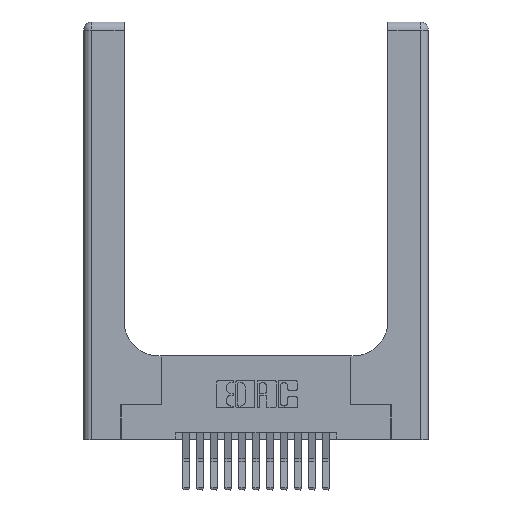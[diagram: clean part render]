
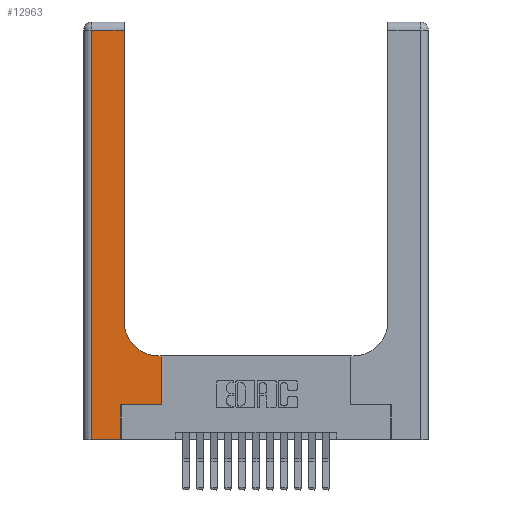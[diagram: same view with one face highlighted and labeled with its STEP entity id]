
A CAD part, top view. The second image highlights one B-rep face of the part: STEP entity #12963.
In plain terms, the highlighted planar face has unit normal (0, 0, 1).
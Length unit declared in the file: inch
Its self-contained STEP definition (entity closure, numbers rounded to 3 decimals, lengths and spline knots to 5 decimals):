
#119 = ORIENTED_EDGE ( 'NONE', *, *, #17524, .T. ) ;
#681 = ORIENTED_EDGE ( 'NONE', *, *, #6312, .T. ) ;
#894 = CARTESIAN_POINT ( 'NONE',  ( 0.5585, 0.6, 0.37 ) ) ;
#912 = LINE ( 'NONE', #16694, #14857 ) ;
#940 = EDGE_CURVE ( 'NONE', #12710, #9015, #12921, .T. ) ;
#1045 = AXIS2_PLACEMENT_3D ( 'NONE', #9175, #6428, #3822 ) ;
#1294 = EDGE_CURVE ( 'NONE', #9015, #9551, #13995, .T. ) ;
#1590 = CARTESIAN_POINT ( 'NONE',  ( 0.5415, 0.85, 0.37 ) ) ;
#1810 = LINE ( 'NONE', #12224, #9227 ) ;
#2588 = CARTESIAN_POINT ( 'NONE',  ( 0.5585, 0.25, 0.37 ) ) ;
#2897 = CARTESIAN_POINT ( 'NONE',  ( 0.2915, 2.94, 0.37 ) ) ;
#3028 = VECTOR ( 'NONE', #9323, 39.37008 ) ;
#3314 = CIRCLE ( 'NONE', #15575, 0.25 ) ;
#3367 = CARTESIAN_POINT ( 'NONE',  ( 0.5585, 0.25, 0.37 ) ) ;
#3822 = DIRECTION ( 'NONE',  ( -1., 0., 0. ) ) ;
#4126 = ORIENTED_EDGE ( 'NONE', *, *, #7134, .T. ) ;
#4908 = DIRECTION ( 'NONE',  ( 0., 1., 0. ) ) ;
#5151 = ORIENTED_EDGE ( 'NONE', *, *, #17037, .T. ) ;
#5170 = ORIENTED_EDGE ( 'NONE', *, *, #13499, .T. ) ;
#5340 = LINE ( 'NONE', #11966, #11842 ) ;
#5417 = DIRECTION ( 'NONE',  ( -1., 0., 0. ) ) ;
#5501 = ORIENTED_EDGE ( 'NONE', *, *, #17718, .T. ) ;
#5720 = ORIENTED_EDGE ( 'NONE', *, *, #14791, .T. ) ;
#6036 = CARTESIAN_POINT ( 'NONE',  ( 0.06, 2.94, 0.37 ) ) ;
#6074 = DIRECTION ( 'NONE',  ( 1., 0., 0. ) ) ;
#6312 = EDGE_CURVE ( 'NONE', #15978, #18007, #1810, .T. ) ;
#6428 = DIRECTION ( 'NONE',  ( 0., 0., -1. ) ) ;
#6876 = VECTOR ( 'NONE', #13115, 39.37008 ) ;
#7134 = EDGE_CURVE ( 'NONE', #9644, #15978, #3314, .T. ) ;
#7175 = DIRECTION ( 'NONE',  ( 1., 0., 0. ) ) ;
#7241 = CARTESIAN_POINT ( 'NONE',  ( 0.269, 0., 0.37 ) ) ;
#7255 = ORIENTED_EDGE ( 'NONE', *, *, #1294, .T. ) ;
#7330 = VERTEX_POINT ( 'NONE', #7241 ) ;
#8597 = VECTOR ( 'NONE', #11165, 39.37008 ) ;
#8750 = VERTEX_POINT ( 'NONE', #16510 ) ;
#9015 = VERTEX_POINT ( 'NONE', #2588 ) ;
#9175 = CARTESIAN_POINT ( 'NONE',  ( 0., 3., 0.37 ) ) ;
#9227 = VECTOR ( 'NONE', #15043, 39.37008 ) ;
#9323 = DIRECTION ( 'NONE',  ( 0., -1., 0. ) ) ;
#9399 = ORIENTED_EDGE ( 'NONE', *, *, #940, .T. ) ;
#9551 = VERTEX_POINT ( 'NONE', #894 ) ;
#9644 = VERTEX_POINT ( 'NONE', #13931 ) ;
#10290 = FACE_OUTER_BOUND ( 'NONE', #15861, .T. ) ;
#10336 = CARTESIAN_POINT ( 'NONE',  ( 0., 2.94, 0.37 ) ) ;
#10959 = VECTOR ( 'NONE', #6074, 39.37008 ) ;
#11165 = DIRECTION ( 'NONE',  ( 1., 0., 0. ) ) ;
#11301 = DIRECTION ( 'NONE',  ( 0., 0., -1. ) ) ;
#11791 = CARTESIAN_POINT ( 'NONE',  ( 0., 0., 0.37 ) ) ;
#11842 = VECTOR ( 'NONE', #5417, 39.37008 ) ;
#11966 = CARTESIAN_POINT ( 'NONE',  ( 0.2915, 0.6, 0.37 ) ) ;
#12224 = CARTESIAN_POINT ( 'NONE',  ( 0.2915, 3., 0.37 ) ) ;
#12627 = CARTESIAN_POINT ( 'NONE',  ( 0.269, 0.25, 0.37 ) ) ;
#12710 = VERTEX_POINT ( 'NONE', #17160 ) ;
#12921 = LINE ( 'NONE', #12627, #8597 ) ;
#12963 = ADVANCED_FACE ( 'NONE', ( #10290 ), #17533, .F. ) ;
#13115 = DIRECTION ( 'NONE',  ( -1., 0., 0. ) ) ;
#13380 = CARTESIAN_POINT ( 'NONE',  ( 0.06, 3., 0.37 ) ) ;
#13499 = EDGE_CURVE ( 'NONE', #7330, #12710, #912, .T. ) ;
#13931 = CARTESIAN_POINT ( 'NONE',  ( 0.5415, 0.6, 0.37 ) ) ;
#13995 = LINE ( 'NONE', #3367, #17311 ) ;
#14106 = LINE ( 'NONE', #13380, #3028 ) ;
#14467 = LINE ( 'NONE', #11791, #10959 ) ;
#14601 = VERTEX_POINT ( 'NONE', #6036 ) ;
#14791 = EDGE_CURVE ( 'NONE', #14601, #8750, #14106, .T. ) ;
#14857 = VECTOR ( 'NONE', #15046, 39.37008 ) ;
#15043 = DIRECTION ( 'NONE',  ( 0., 1., 0. ) ) ;
#15046 = DIRECTION ( 'NONE',  ( 0., 1., 0. ) ) ;
#15575 = AXIS2_PLACEMENT_3D ( 'NONE', #1590, #11301, #7175 ) ;
#15861 = EDGE_LOOP ( 'NONE', ( #681, #5151, #5720, #119, #5170, #9399, #7255, #5501, #4126 ) ) ;
#15978 = VERTEX_POINT ( 'NONE', #15986 ) ;
#15986 = CARTESIAN_POINT ( 'NONE',  ( 0.2915, 0.85, 0.37 ) ) ;
#16455 = LINE ( 'NONE', #10336, #6876 ) ;
#16510 = CARTESIAN_POINT ( 'NONE',  ( 0.06, 0., 0.37 ) ) ;
#16694 = CARTESIAN_POINT ( 'NONE',  ( 0.269, 0., 0.37 ) ) ;
#17037 = EDGE_CURVE ( 'NONE', #18007, #14601, #16455, .T. ) ;
#17160 = CARTESIAN_POINT ( 'NONE',  ( 0.269, 0.25, 0.37 ) ) ;
#17311 = VECTOR ( 'NONE', #4908, 39.37008 ) ;
#17524 = EDGE_CURVE ( 'NONE', #8750, #7330, #14467, .T. ) ;
#17533 = PLANE ( 'NONE',  #1045 ) ;
#17718 = EDGE_CURVE ( 'NONE', #9551, #9644, #5340, .T. ) ;
#18007 = VERTEX_POINT ( 'NONE', #2897 ) ;
